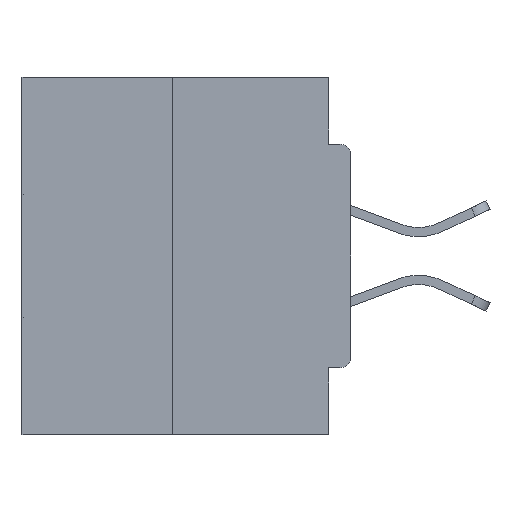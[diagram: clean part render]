
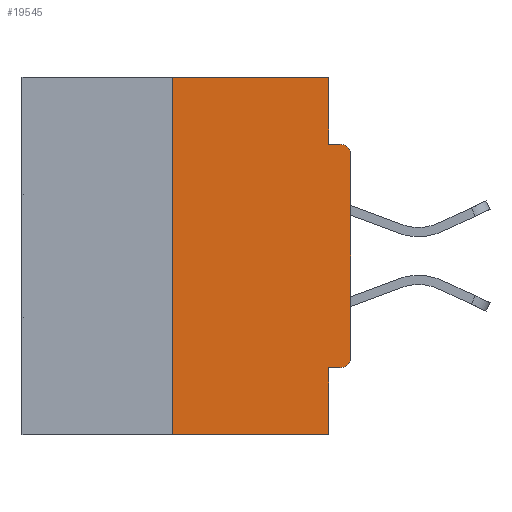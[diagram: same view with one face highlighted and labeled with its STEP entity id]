
A CAD part, left-side view. The second image highlights one B-rep face of the part: STEP entity #19545.
In plain terms, the highlighted planar face has unit normal (-1, 0, 0).
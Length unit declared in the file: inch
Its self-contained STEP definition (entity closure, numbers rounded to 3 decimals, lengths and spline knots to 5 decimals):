
#469 = ORIENTED_EDGE ( 'NONE', *, *, #26219, .F. ) ;
#533 = VERTEX_POINT ( 'NONE', #3077 ) ;
#884 = DIRECTION ( 'NONE',  ( 0., 0., -1. ) ) ;
#890 = CARTESIAN_POINT ( 'NONE',  ( 0., 0.015, -0.1085 ) ) ;
#971 = DIRECTION ( 'NONE',  ( 0., 0., 1. ) ) ;
#1227 = CARTESIAN_POINT ( 'NONE',  ( 0., 0.25, -0.5 ) ) ;
#1271 = EDGE_CURVE ( 'NONE', #8116, #19513, #32410, .T. ) ;
#1360 = DIRECTION ( 'NONE',  ( 0., 0., -1. ) ) ;
#1493 = CIRCLE ( 'NONE', #24641, 0.015 ) ;
#2162 = LINE ( 'NONE', #20102, #5097 ) ;
#2204 = CARTESIAN_POINT ( 'NONE',  ( 0., 0., -0.3915 ) ) ;
#2328 = EDGE_CURVE ( 'NONE', #23970, #8262, #15284, .T. ) ;
#2950 = EDGE_CURVE ( 'NONE', #16858, #23970, #2162, .T. ) ;
#3077 = CARTESIAN_POINT ( 'NONE',  ( 0., 0.015, -0.4065 ) ) ;
#3168 = CARTESIAN_POINT ( 'NONE',  ( 0., 0.031, -0.4065 ) ) ;
#4434 = DIRECTION ( 'NONE',  ( -1., 0., 0. ) ) ;
#4491 = CARTESIAN_POINT ( 'NONE',  ( 0., 0., -0.1085 ) ) ;
#4835 = CARTESIAN_POINT ( 'NONE',  ( 0., 0.46, -0.5 ) ) ;
#5097 = VECTOR ( 'NONE', #1360, 39.37008 ) ;
#5736 = VECTOR ( 'NONE', #14982, 39.37008 ) ;
#7021 = ORIENTED_EDGE ( 'NONE', *, *, #29406, .F. ) ;
#8116 = VERTEX_POINT ( 'NONE', #1227 ) ;
#8262 = VERTEX_POINT ( 'NONE', #39540 ) ;
#8276 = ORIENTED_EDGE ( 'NONE', *, *, #2950, .F. ) ;
#9131 = LINE ( 'NONE', #11896, #5736 ) ;
#9383 = VECTOR ( 'NONE', #29440, 39.37008 ) ;
#10651 = CARTESIAN_POINT ( 'NONE',  ( 0., 0.031, -0.0935 ) ) ;
#10821 = DIRECTION ( 'NONE',  ( 0., 0., -1. ) ) ;
#11006 = EDGE_CURVE ( 'NONE', #19321, #19513, #28625, .T. ) ;
#11223 = ORIENTED_EDGE ( 'NONE', *, *, #2328, .F. ) ;
#11368 = CARTESIAN_POINT ( 'NONE',  ( 0., 0., -0.4065 ) ) ;
#11896 = CARTESIAN_POINT ( 'NONE',  ( 0., 0.46, 0. ) ) ;
#13122 = VERTEX_POINT ( 'NONE', #4491 ) ;
#13579 = CARTESIAN_POINT ( 'NONE',  ( 0., 0., 0. ) ) ;
#13978 = EDGE_CURVE ( 'NONE', #533, #40058, #1493, .T. ) ;
#14262 = VECTOR ( 'NONE', #971, 39.37008 ) ;
#14323 = PLANE ( 'NONE',  #17723 ) ;
#14509 = FACE_OUTER_BOUND ( 'NONE', #15761, .T. ) ;
#14982 = DIRECTION ( 'NONE',  ( 0., -1., 0. ) ) ;
#15284 = LINE ( 'NONE', #26000, #24056 ) ;
#15411 = DIRECTION ( 'NONE',  ( 0., 0., 1. ) ) ;
#15761 = EDGE_LOOP ( 'NONE', ( #32065, #7021, #26879, #36369, #469, #40069, #37687, #37696, #11223, #8276 ) ) ;
#16469 = CIRCLE ( 'NONE', #32937, 0.015 ) ;
#16858 = VERTEX_POINT ( 'NONE', #19008 ) ;
#17579 = LINE ( 'NONE', #11368, #9383 ) ;
#17723 = AXIS2_PLACEMENT_3D ( 'NONE', #20220, #33061, #26685 ) ;
#19008 = CARTESIAN_POINT ( 'NONE',  ( 0., 0.031, 0. ) ) ;
#19321 = VERTEX_POINT ( 'NONE', #3168 ) ;
#19481 = CARTESIAN_POINT ( 'NONE',  ( 0., 0.015, -0.3915 ) ) ;
#19513 = VERTEX_POINT ( 'NONE', #32293 ) ;
#19545 = ADVANCED_FACE ( 'NONE', ( #14509 ), #14323, .F. ) ;
#20102 = CARTESIAN_POINT ( 'NONE',  ( 0., 0.031, 0. ) ) ;
#20220 = CARTESIAN_POINT ( 'NONE',  ( 0., 0.46, 0. ) ) ;
#20911 = CARTESIAN_POINT ( 'NONE',  ( 0., 0.25, 0. ) ) ;
#21807 = CARTESIAN_POINT ( 'NONE',  ( 0., 0.25, 0. ) ) ;
#22644 = VERTEX_POINT ( 'NONE', #20911 ) ;
#22785 = VECTOR ( 'NONE', #38166, 39.37008 ) ;
#23970 = VERTEX_POINT ( 'NONE', #10651 ) ;
#24056 = VECTOR ( 'NONE', #35745, 39.37008 ) ;
#24641 = AXIS2_PLACEMENT_3D ( 'NONE', #19481, #28734, #884 ) ;
#25116 = VECTOR ( 'NONE', #15411, 39.37008 ) ;
#26000 = CARTESIAN_POINT ( 'NONE',  ( 0., 0., -0.0935 ) ) ;
#26219 = EDGE_CURVE ( 'NONE', #533, #19321, #17579, .T. ) ;
#26517 = DIRECTION ( 'NONE',  ( 0., -1., 0. ) ) ;
#26685 = DIRECTION ( 'NONE',  ( 0., 0., -1. ) ) ;
#26879 = ORIENTED_EDGE ( 'NONE', *, *, #1271, .T. ) ;
#28594 = CARTESIAN_POINT ( 'NONE',  ( 0., 0.031, -0.5 ) ) ;
#28625 = LINE ( 'NONE', #28594, #22785 ) ;
#28734 = DIRECTION ( 'NONE',  ( -1., 0., 0. ) ) ;
#29406 = EDGE_CURVE ( 'NONE', #8116, #22644, #37242, .T. ) ;
#29440 = DIRECTION ( 'NONE',  ( 0., 1., 0. ) ) ;
#31182 = EDGE_CURVE ( 'NONE', #13122, #8262, #16469, .T. ) ;
#32065 = ORIENTED_EDGE ( 'NONE', *, *, #32363, .F. ) ;
#32293 = CARTESIAN_POINT ( 'NONE',  ( 0., 0.031, -0.5 ) ) ;
#32363 = EDGE_CURVE ( 'NONE', #22644, #16858, #9131, .T. ) ;
#32410 = LINE ( 'NONE', #4835, #37718 ) ;
#32746 = LINE ( 'NONE', #13579, #14262 ) ;
#32937 = AXIS2_PLACEMENT_3D ( 'NONE', #890, #4434, #10821 ) ;
#33061 = DIRECTION ( 'NONE',  ( 1., 0., 0. ) ) ;
#34104 = EDGE_CURVE ( 'NONE', #40058, #13122, #32746, .T. ) ;
#35745 = DIRECTION ( 'NONE',  ( 0., -1., 0. ) ) ;
#36369 = ORIENTED_EDGE ( 'NONE', *, *, #11006, .F. ) ;
#37242 = LINE ( 'NONE', #21807, #25116 ) ;
#37687 = ORIENTED_EDGE ( 'NONE', *, *, #34104, .T. ) ;
#37696 = ORIENTED_EDGE ( 'NONE', *, *, #31182, .T. ) ;
#37718 = VECTOR ( 'NONE', #26517, 39.37008 ) ;
#38166 = DIRECTION ( 'NONE',  ( 0., 0., -1. ) ) ;
#39540 = CARTESIAN_POINT ( 'NONE',  ( 0., 0.015, -0.0935 ) ) ;
#40058 = VERTEX_POINT ( 'NONE', #2204 ) ;
#40069 = ORIENTED_EDGE ( 'NONE', *, *, #13978, .T. ) ;
